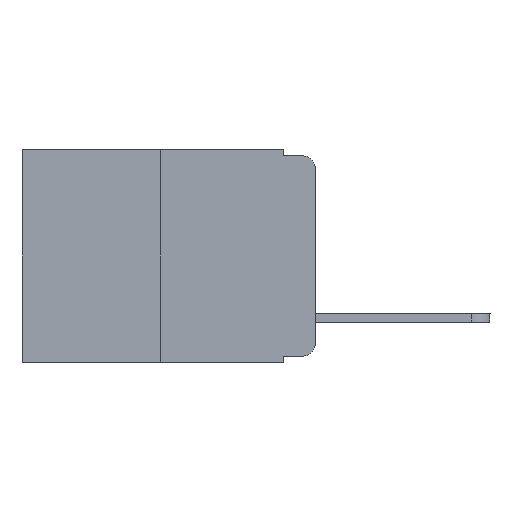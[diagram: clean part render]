
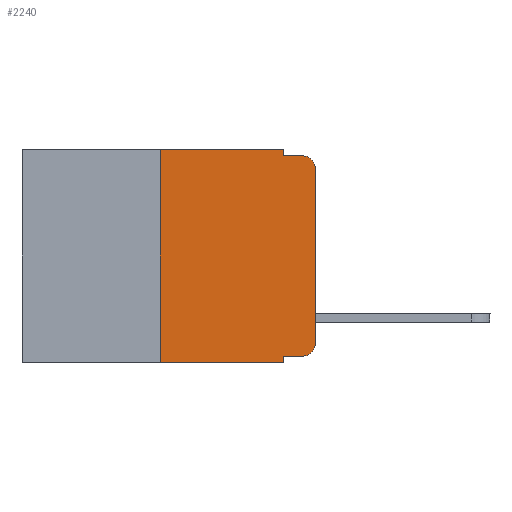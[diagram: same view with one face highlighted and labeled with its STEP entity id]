
A CAD part, left-side view. The second image highlights one B-rep face of the part: STEP entity #2240.
In plain terms, the highlighted planar face has unit normal (-1, 0, 0).
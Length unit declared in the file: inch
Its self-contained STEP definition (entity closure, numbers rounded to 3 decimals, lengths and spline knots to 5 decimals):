
#199 = EDGE_CURVE ( 'NONE', #10269, #21190, #14996, .T. ) ;
#636 = ORIENTED_EDGE ( 'NONE', *, *, #7658, .F. ) ;
#707 = CARTESIAN_POINT ( 'NONE',  ( 0., 0.051, 0. ) ) ;
#761 = ORIENTED_EDGE ( 'NONE', *, *, #24290, .F. ) ;
#1071 = DIRECTION ( 'NONE',  ( 0., 0., -1. ) ) ;
#1475 = EDGE_CURVE ( 'NONE', #10269, #20177, #16514, .T. ) ;
#1838 = EDGE_CURVE ( 'NONE', #15638, #5504, #10198, .T. ) ;
#2096 = ORIENTED_EDGE ( 'NONE', *, *, #3990, .T. ) ;
#2240 = ADVANCED_FACE ( 'NONE', ( #10431 ), #23918, .F. ) ;
#2573 = LINE ( 'NONE', #14223, #8589 ) ;
#2702 = DIRECTION ( 'NONE',  ( 0., 0., 1. ) ) ;
#3760 = LINE ( 'NONE', #3888, #10682 ) ;
#3888 = CARTESIAN_POINT ( 'NONE',  ( 0., 0.051, -0.01 ) ) ;
#3990 = EDGE_CURVE ( 'NONE', #13587, #15638, #20235, .T. ) ;
#4427 = CARTESIAN_POINT ( 'NONE',  ( 0., 0.02, -0.01 ) ) ;
#4510 = CARTESIAN_POINT ( 'NONE',  ( 0., 0.02, -0.03 ) ) ;
#4689 = LINE ( 'NONE', #15821, #19006 ) ;
#5403 = VERTEX_POINT ( 'NONE', #23246 ) ;
#5491 = CARTESIAN_POINT ( 'NONE',  ( 0., 0.473, -0.343 ) ) ;
#5504 = VERTEX_POINT ( 'NONE', #4427 ) ;
#6457 = VECTOR ( 'NONE', #22905, 39.37008 ) ;
#6513 = DIRECTION ( 'NONE',  ( -1., 0., 0. ) ) ;
#6832 = ORIENTED_EDGE ( 'NONE', *, *, #21144, .F. ) ;
#6863 = CARTESIAN_POINT ( 'NONE',  ( 0., 0., 0. ) ) ;
#7436 = VECTOR ( 'NONE', #1071, 39.37008 ) ;
#7658 = EDGE_CURVE ( 'NONE', #20451, #5403, #4689, .T. ) ;
#7753 = CARTESIAN_POINT ( 'NONE',  ( 0., 0.051, -0.333 ) ) ;
#7769 = CARTESIAN_POINT ( 'NONE',  ( 0., 0.25, -0.343 ) ) ;
#8271 = ORIENTED_EDGE ( 'NONE', *, *, #24750, .T. ) ;
#8465 = VECTOR ( 'NONE', #8942, 39.37008 ) ;
#8467 = DIRECTION ( 'NONE',  ( 0., 0., -1. ) ) ;
#8548 = ORIENTED_EDGE ( 'NONE', *, *, #1838, .T. ) ;
#8589 = VECTOR ( 'NONE', #2702, 39.37008 ) ;
#8710 = DIRECTION ( 'NONE',  ( 0., 0., -1. ) ) ;
#8942 = DIRECTION ( 'NONE',  ( 0., -1., 0. ) ) ;
#9202 = CARTESIAN_POINT ( 'NONE',  ( 0., 0.051, -0.333 ) ) ;
#9830 = AXIS2_PLACEMENT_3D ( 'NONE', #14100, #21524, #11946 ) ;
#10022 = EDGE_CURVE ( 'NONE', #19845, #5504, #3760, .T. ) ;
#10198 = CIRCLE ( 'NONE', #11406, 0.02 ) ;
#10269 = VERTEX_POINT ( 'NONE', #7753 ) ;
#10431 = FACE_OUTER_BOUND ( 'NONE', #11285, .T. ) ;
#10682 = VECTOR ( 'NONE', #15395, 39.37008 ) ;
#11285 = EDGE_LOOP ( 'NONE', ( #2096, #8548, #19405, #761, #636, #6832, #14507, #17312, #23998, #8271 ) ) ;
#11406 = AXIS2_PLACEMENT_3D ( 'NONE', #4510, #24081, #8710 ) ;
#11946 = DIRECTION ( 'NONE',  ( 0., 0., -1. ) ) ;
#12029 = DIRECTION ( 'NONE',  ( 0., -1., 0. ) ) ;
#13587 = VERTEX_POINT ( 'NONE', #17977 ) ;
#14100 = CARTESIAN_POINT ( 'NONE',  ( 0., 0.473, 0. ) ) ;
#14223 = CARTESIAN_POINT ( 'NONE',  ( 0., 0.25, 0. ) ) ;
#14233 = DIRECTION ( 'NONE',  ( 0., 0., -1. ) ) ;
#14507 = ORIENTED_EDGE ( 'NONE', *, *, #17253, .T. ) ;
#14774 = VECTOR ( 'NONE', #22251, 39.37008 ) ;
#14996 = LINE ( 'NONE', #9202, #8465 ) ;
#15395 = DIRECTION ( 'NONE',  ( 0., -1., 0. ) ) ;
#15638 = VERTEX_POINT ( 'NONE', #19238 ) ;
#15821 = CARTESIAN_POINT ( 'NONE',  ( 0., 0.473, 0. ) ) ;
#16514 = LINE ( 'NONE', #24314, #7436 ) ;
#16610 = CARTESIAN_POINT ( 'NONE',  ( 0., 0.02, -0.333 ) ) ;
#17253 = EDGE_CURVE ( 'NONE', #21879, #20177, #18994, .T. ) ;
#17312 = ORIENTED_EDGE ( 'NONE', *, *, #1475, .F. ) ;
#17977 = CARTESIAN_POINT ( 'NONE',  ( 0., 0., -0.313 ) ) ;
#18054 = LINE ( 'NONE', #707, #24350 ) ;
#18994 = LINE ( 'NONE', #5491, #6457 ) ;
#19006 = VECTOR ( 'NONE', #12029, 39.37008 ) ;
#19050 = CARTESIAN_POINT ( 'NONE',  ( 0., 0.25, 0. ) ) ;
#19238 = CARTESIAN_POINT ( 'NONE',  ( 0., 0., -0.03 ) ) ;
#19405 = ORIENTED_EDGE ( 'NONE', *, *, #10022, .F. ) ;
#19845 = VERTEX_POINT ( 'NONE', #22268 ) ;
#20177 = VERTEX_POINT ( 'NONE', #21739 ) ;
#20235 = LINE ( 'NONE', #6863, #14774 ) ;
#20352 = CIRCLE ( 'NONE', #23164, 0.02 ) ;
#20451 = VERTEX_POINT ( 'NONE', #19050 ) ;
#21144 = EDGE_CURVE ( 'NONE', #21879, #20451, #2573, .T. ) ;
#21190 = VERTEX_POINT ( 'NONE', #16610 ) ;
#21524 = DIRECTION ( 'NONE',  ( 1., 0., 0. ) ) ;
#21739 = CARTESIAN_POINT ( 'NONE',  ( 0., 0.051, -0.343 ) ) ;
#21879 = VERTEX_POINT ( 'NONE', #7769 ) ;
#22251 = DIRECTION ( 'NONE',  ( 0., 0., 1. ) ) ;
#22268 = CARTESIAN_POINT ( 'NONE',  ( 0., 0.051, -0.01 ) ) ;
#22905 = DIRECTION ( 'NONE',  ( 0., -1., 0. ) ) ;
#23164 = AXIS2_PLACEMENT_3D ( 'NONE', #23804, #6513, #14233 ) ;
#23246 = CARTESIAN_POINT ( 'NONE',  ( 0., 0.051, 0. ) ) ;
#23804 = CARTESIAN_POINT ( 'NONE',  ( 0., 0.02, -0.313 ) ) ;
#23918 = PLANE ( 'NONE',  #9830 ) ;
#23998 = ORIENTED_EDGE ( 'NONE', *, *, #199, .T. ) ;
#24081 = DIRECTION ( 'NONE',  ( -1., 0., 0. ) ) ;
#24290 = EDGE_CURVE ( 'NONE', #5403, #19845, #18054, .T. ) ;
#24314 = CARTESIAN_POINT ( 'NONE',  ( 0., 0.051, 0. ) ) ;
#24350 = VECTOR ( 'NONE', #8467, 39.37008 ) ;
#24750 = EDGE_CURVE ( 'NONE', #21190, #13587, #20352, .T. ) ;
